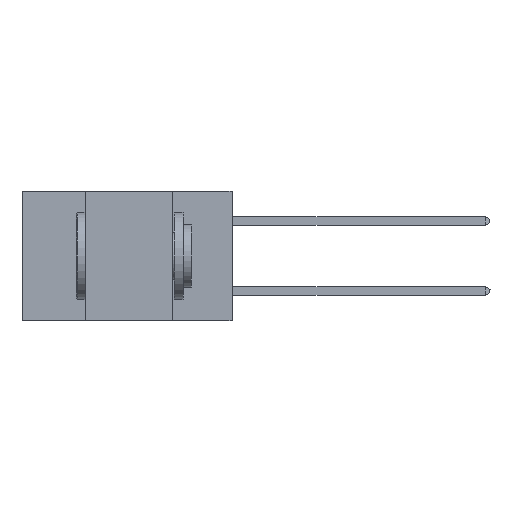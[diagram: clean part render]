
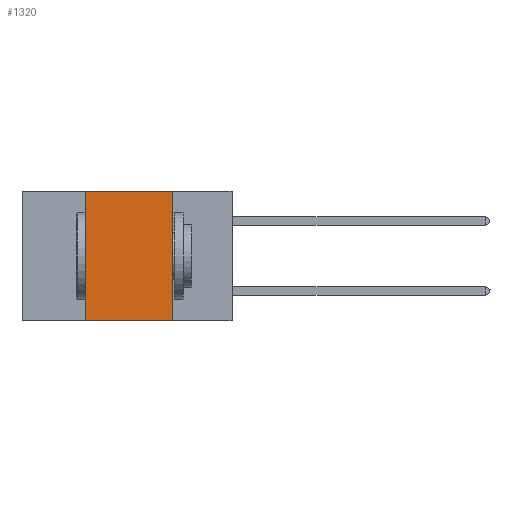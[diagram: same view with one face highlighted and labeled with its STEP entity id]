
A CAD part, left-side view. The second image highlights one B-rep face of the part: STEP entity #1320.
In plain terms, the highlighted planar face has unit normal (-1, 0, 0).
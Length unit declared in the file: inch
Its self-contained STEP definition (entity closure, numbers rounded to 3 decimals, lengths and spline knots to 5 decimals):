
#1320 = ADVANCED_FACE ( 'NONE', ( #5424 ), #32390, .F. ) ;
#4108 = EDGE_CURVE ( 'NONE', #17254, #15934, #34063, .T. ) ;
#4322 = CARTESIAN_POINT ( 'NONE',  ( 0., 0.6, -0.37 ) ) ;
#5424 = FACE_OUTER_BOUND ( 'NONE', #32365, .T. ) ;
#5580 = CARTESIAN_POINT ( 'NONE',  ( 0., 0.17, 0. ) ) ;
#7761 = DIRECTION ( 'NONE',  ( 1., 0., 0. ) ) ;
#8188 = LINE ( 'NONE', #13021, #24681 ) ;
#9085 = LINE ( 'NONE', #4322, #14573 ) ;
#11930 = DIRECTION ( 'NONE',  ( 0., -1., 0. ) ) ;
#13021 = CARTESIAN_POINT ( 'NONE',  ( 0., 0.42, 0. ) ) ;
#13133 = DIRECTION ( 'NONE',  ( 0., 0., -1. ) ) ;
#13688 = CARTESIAN_POINT ( 'NONE',  ( 0., 0.42, 0. ) ) ;
#14136 = VECTOR ( 'NONE', #34527, 39.37008 ) ;
#14193 = EDGE_CURVE ( 'NONE', #15934, #34429, #22557, .T. ) ;
#14573 = VECTOR ( 'NONE', #11930, 39.37008 ) ;
#15480 = CARTESIAN_POINT ( 'NONE',  ( 0., 0.17, 0. ) ) ;
#15934 = VERTEX_POINT ( 'NONE', #5580 ) ;
#17254 = VERTEX_POINT ( 'NONE', #13688 ) ;
#17468 = VECTOR ( 'NONE', #13133, 39.37008 ) ;
#18264 = CARTESIAN_POINT ( 'NONE',  ( 0., 0.42, -0.37 ) ) ;
#18766 = CARTESIAN_POINT ( 'NONE',  ( 0., 0.6, 0. ) ) ;
#19749 = AXIS2_PLACEMENT_3D ( 'NONE', #18766, #7761, #32156 ) ;
#21100 = EDGE_CURVE ( 'NONE', #28996, #34429, #9085, .T. ) ;
#22361 = EDGE_CURVE ( 'NONE', #28996, #17254, #8188, .T. ) ;
#22557 = LINE ( 'NONE', #15480, #17468 ) ;
#23866 = CARTESIAN_POINT ( 'NONE',  ( 0., 0.6, 0. ) ) ;
#24681 = VECTOR ( 'NONE', #26912, 39.37008 ) ;
#26361 = ORIENTED_EDGE ( 'NONE', *, *, #4108, .F. ) ;
#26597 = ORIENTED_EDGE ( 'NONE', *, *, #21100, .T. ) ;
#26732 = CARTESIAN_POINT ( 'NONE',  ( 0., 0.17, -0.37 ) ) ;
#26912 = DIRECTION ( 'NONE',  ( 0., 0., 1. ) ) ;
#27671 = ORIENTED_EDGE ( 'NONE', *, *, #22361, .F. ) ;
#28996 = VERTEX_POINT ( 'NONE', #18264 ) ;
#31265 = ORIENTED_EDGE ( 'NONE', *, *, #14193, .F. ) ;
#32156 = DIRECTION ( 'NONE',  ( 0., 0., -1. ) ) ;
#32365 = EDGE_LOOP ( 'NONE', ( #31265, #26361, #27671, #26597 ) ) ;
#32390 = PLANE ( 'NONE',  #19749 ) ;
#34063 = LINE ( 'NONE', #23866, #14136 ) ;
#34429 = VERTEX_POINT ( 'NONE', #26732 ) ;
#34527 = DIRECTION ( 'NONE',  ( 0., -1., 0. ) ) ;
